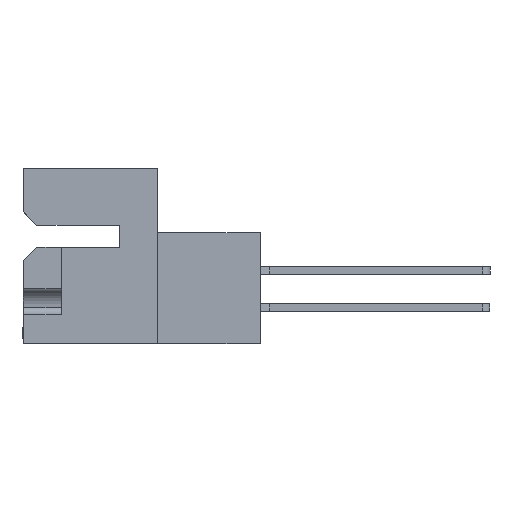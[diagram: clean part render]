
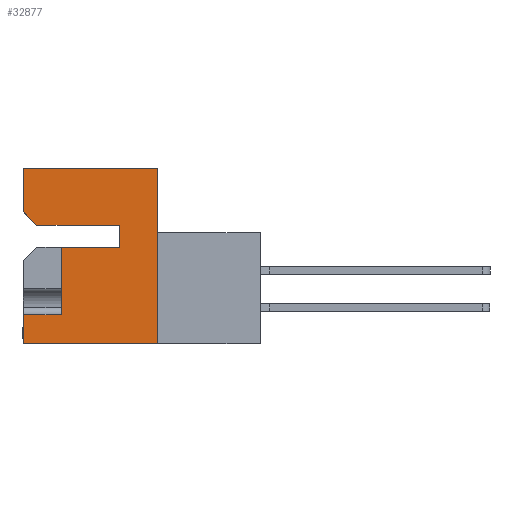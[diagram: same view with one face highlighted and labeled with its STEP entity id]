
A CAD part, left-side view. The second image highlights one B-rep face of the part: STEP entity #32877.
In plain terms, the highlighted planar face has unit normal (-1, 0, 0).
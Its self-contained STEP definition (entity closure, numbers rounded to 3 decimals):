
#299 = DIRECTION ( 'NONE',  ( 0., 1., 0. ) ) ;
#751 = LINE ( 'NONE', #17520, #35679 ) ;
#1183 = CARTESIAN_POINT ( 'NONE',  ( 0., 0., 0. ) ) ;
#2126 = ORIENTED_EDGE ( 'NONE', *, *, #16132, .F. ) ;
#2314 = EDGE_CURVE ( 'NONE', #44916, #6323, #51602, .T. ) ;
#2414 = DIRECTION ( 'NONE',  ( 0., 1., 0. ) ) ;
#2569 = ORIENTED_EDGE ( 'NONE', *, *, #9219, .T. ) ;
#3549 = CARTESIAN_POINT ( 'NONE',  ( 0., -8.814, -15.088 ) ) ;
#3660 = ORIENTED_EDGE ( 'NONE', *, *, #7759, .F. ) ;
#4911 = LINE ( 'NONE', #43026, #51143 ) ;
#5210 = CARTESIAN_POINT ( 'NONE',  ( 0., 3.251, -6.782 ) ) ;
#5815 = CARTESIAN_POINT ( 'NONE',  ( 0., 11.506, -3.759 ) ) ;
#6132 = DIRECTION ( 'NONE',  ( 0., -1., 0. ) ) ;
#6323 = VERTEX_POINT ( 'NONE', #48072 ) ;
#6497 = VERTEX_POINT ( 'NONE', #5815 ) ;
#7526 = EDGE_CURVE ( 'NONE', #43738, #21874, #37595, .T. ) ;
#7759 = EDGE_CURVE ( 'NONE', #18909, #44916, #28178, .T. ) ;
#7880 = CARTESIAN_POINT ( 'NONE',  ( 0., 3.251, -6.782 ) ) ;
#8095 = VECTOR ( 'NONE', #9036, 1000. ) ;
#8737 = DIRECTION ( 'NONE',  ( 0., 0., 1. ) ) ;
#9036 = DIRECTION ( 'NONE',  ( 0., -0.707, -0.707 ) ) ;
#9219 = EDGE_CURVE ( 'NONE', #6497, #15151, #45514, .T. ) ;
#9545 = PLANE ( 'NONE',  #34380 ) ;
#10401 = VECTOR ( 'NONE', #10997, 1000. ) ;
#10672 = DIRECTION ( 'NONE',  ( 0., 0., 1. ) ) ;
#10766 = VECTOR ( 'NONE', #15060, 1000. ) ;
#10997 = DIRECTION ( 'NONE',  ( 0., 0., -1. ) ) ;
#11316 = VECTOR ( 'NONE', #2414, 1000. ) ;
#14022 = EDGE_LOOP ( 'NONE', ( #49799, #23200, #3660, #30744, #2569, #36228, #49908, #2126, #32277, #31353, #51679 ) ) ;
#15060 = DIRECTION ( 'NONE',  ( 0., 1., 0. ) ) ;
#15151 = VERTEX_POINT ( 'NONE', #49846 ) ;
#16117 = VECTOR ( 'NONE', #27257, 1000. ) ;
#16132 = EDGE_CURVE ( 'NONE', #43837, #51631, #751, .T. ) ;
#16324 = LINE ( 'NONE', #38527, #11316 ) ;
#17130 = DIRECTION ( 'NONE',  ( 0., 0., 1. ) ) ;
#17520 = CARTESIAN_POINT ( 'NONE',  ( 0., 0., -6.782 ) ) ;
#17901 = EDGE_CURVE ( 'NONE', #21509, #15151, #16324, .T. ) ;
#17943 = VECTOR ( 'NONE', #10672, 1000. ) ;
#18505 = VECTOR ( 'NONE', #17130, 1000. ) ;
#18909 = VERTEX_POINT ( 'NONE', #49429 ) ;
#18944 = VECTOR ( 'NONE', #8737, 1000. ) ;
#18970 = FACE_OUTER_BOUND ( 'NONE', #14022, .T. ) ;
#19116 = VERTEX_POINT ( 'NONE', #42074 ) ;
#21509 = VERTEX_POINT ( 'NONE', #27700 ) ;
#21874 = VERTEX_POINT ( 'NONE', #39402 ) ;
#23200 = ORIENTED_EDGE ( 'NONE', *, *, #2314, .F. ) ;
#23884 = LINE ( 'NONE', #3549, #10766 ) ;
#25746 = DIRECTION ( 'NONE',  ( 1., 0., 0. ) ) ;
#26766 = EDGE_CURVE ( 'NONE', #19116, #21874, #4911, .T. ) ;
#27257 = DIRECTION ( 'NONE',  ( 0., 0., 1. ) ) ;
#27700 = CARTESIAN_POINT ( 'NONE',  ( 0., 3.251, -4.902 ) ) ;
#27781 = EDGE_CURVE ( 'NONE', #19116, #43837, #29164, .T. ) ;
#28178 = LINE ( 'NONE', #35300, #47596 ) ;
#29164 = LINE ( 'NONE', #51176, #16117 ) ;
#30744 = ORIENTED_EDGE ( 'NONE', *, *, #42046, .F. ) ;
#31353 = ORIENTED_EDGE ( 'NONE', *, *, #26766, .T. ) ;
#31519 = EDGE_CURVE ( 'NONE', #6323, #43738, #23884, .T. ) ;
#31711 = CARTESIAN_POINT ( 'NONE',  ( 0., 0., 0. ) ) ;
#32277 = ORIENTED_EDGE ( 'NONE', *, *, #27781, .F. ) ;
#32877 = ADVANCED_FACE ( 'NONE', ( #18970 ), #9545, .F. ) ;
#33557 = CARTESIAN_POINT ( 'NONE',  ( 0., 10.363, -4.902 ) ) ;
#33912 = DIRECTION ( 'NONE',  ( 0., 0., -1. ) ) ;
#34380 = AXIS2_PLACEMENT_3D ( 'NONE', #1183, #25746, #33912 ) ;
#35300 = CARTESIAN_POINT ( 'NONE',  ( 0., 11.506, 0. ) ) ;
#35622 = EDGE_CURVE ( 'NONE', #51631, #21509, #41468, .T. ) ;
#35679 = VECTOR ( 'NONE', #6132, 1000. ) ;
#36228 = ORIENTED_EDGE ( 'NONE', *, *, #17901, .F. ) ;
#37595 = LINE ( 'NONE', #44975, #18944 ) ;
#38527 = CARTESIAN_POINT ( 'NONE',  ( 0., 0., -4.902 ) ) ;
#38666 = CARTESIAN_POINT ( 'NONE',  ( 0., 0., 0. ) ) ;
#39084 = LINE ( 'NONE', #50802, #17943 ) ;
#39402 = CARTESIAN_POINT ( 'NONE',  ( 0., 11.506, -12.58 ) ) ;
#41468 = LINE ( 'NONE', #5210, #18505 ) ;
#42046 = EDGE_CURVE ( 'NONE', #6497, #18909, #39084, .T. ) ;
#42074 = CARTESIAN_POINT ( 'NONE',  ( 0., 8.255, -12.58 ) ) ;
#42098 = CARTESIAN_POINT ( 'NONE',  ( 0., 11.506, -15.088 ) ) ;
#42613 = CARTESIAN_POINT ( 'NONE',  ( 0., 8.255, -6.782 ) ) ;
#43026 = CARTESIAN_POINT ( 'NONE',  ( 0., 8.255, -12.58 ) ) ;
#43738 = VERTEX_POINT ( 'NONE', #42098 ) ;
#43837 = VERTEX_POINT ( 'NONE', #42613 ) ;
#44916 = VERTEX_POINT ( 'NONE', #31711 ) ;
#44975 = CARTESIAN_POINT ( 'NONE',  ( 0., 11.506, -15.088 ) ) ;
#45514 = LINE ( 'NONE', #33557, #8095 ) ;
#47596 = VECTOR ( 'NONE', #51215, 1000. ) ;
#48072 = CARTESIAN_POINT ( 'NONE',  ( 0., 0., -15.088 ) ) ;
#49429 = CARTESIAN_POINT ( 'NONE',  ( 0., 11.506, 0. ) ) ;
#49799 = ORIENTED_EDGE ( 'NONE', *, *, #31519, .F. ) ;
#49846 = CARTESIAN_POINT ( 'NONE',  ( 0., 10.363, -4.902 ) ) ;
#49908 = ORIENTED_EDGE ( 'NONE', *, *, #35622, .F. ) ;
#50802 = CARTESIAN_POINT ( 'NONE',  ( 0., 11.506, -15.088 ) ) ;
#51143 = VECTOR ( 'NONE', #299, 1000. ) ;
#51176 = CARTESIAN_POINT ( 'NONE',  ( 0., 8.255, -6.782 ) ) ;
#51215 = DIRECTION ( 'NONE',  ( 0., -1., 0. ) ) ;
#51602 = LINE ( 'NONE', #38666, #10401 ) ;
#51631 = VERTEX_POINT ( 'NONE', #7880 ) ;
#51679 = ORIENTED_EDGE ( 'NONE', *, *, #7526, .F. ) ;
